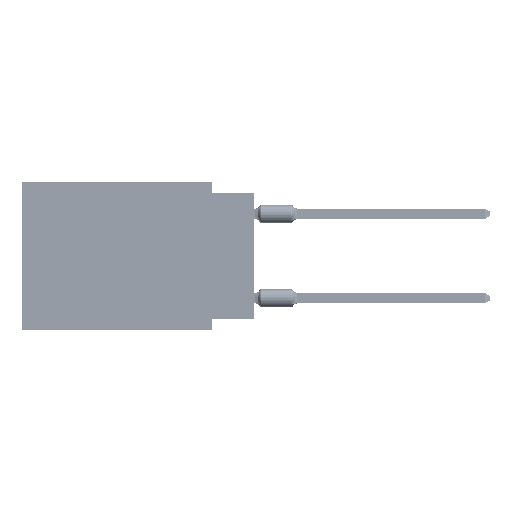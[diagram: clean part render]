
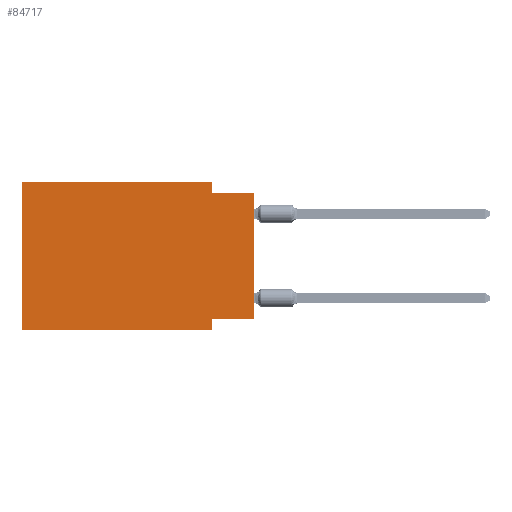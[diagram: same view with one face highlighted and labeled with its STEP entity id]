
A CAD part, left-side view. The second image highlights one B-rep face of the part: STEP entity #84717.
In plain terms, the highlighted planar face has unit normal (-1, 0, 0).
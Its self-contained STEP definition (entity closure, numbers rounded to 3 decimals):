
#614 = CARTESIAN_POINT ( 'NONE',  ( 0., 13.97, 0. ) ) ;
#1731 = DIRECTION ( 'NONE',  ( 0., 0., -1. ) ) ;
#3289 = VERTEX_POINT ( 'NONE', #62890 ) ;
#5989 = ORIENTED_EDGE ( 'NONE', *, *, #31667, .F. ) ;
#6401 = CARTESIAN_POINT ( 'NONE',  ( 0., 0., -0.635 ) ) ;
#9593 = CARTESIAN_POINT ( 'NONE',  ( 0., 0., -8.255 ) ) ;
#10153 = CARTESIAN_POINT ( 'NONE',  ( 0., 13.97, -8.89 ) ) ;
#10672 = LINE ( 'NONE', #44345, #69511 ) ;
#10804 = FACE_OUTER_BOUND ( 'NONE', #86085, .T. ) ;
#12265 = VECTOR ( 'NONE', #18580, 1000. ) ;
#14541 = EDGE_CURVE ( 'NONE', #88609, #100071, #97196, .T. ) ;
#16264 = DIRECTION ( 'NONE',  ( 0., -1., 0. ) ) ;
#18580 = DIRECTION ( 'NONE',  ( 0., -1., 0. ) ) ;
#20111 = CARTESIAN_POINT ( 'NONE',  ( 0., 0., 0. ) ) ;
#23628 = EDGE_CURVE ( 'NONE', #97169, #79795, #48381, .T. ) ;
#24776 = VECTOR ( 'NONE', #54321, 1000. ) ;
#26793 = EDGE_CURVE ( 'NONE', #40394, #40401, #34420, .T. ) ;
#26898 = ORIENTED_EDGE ( 'NONE', *, *, #90787, .F. ) ;
#27081 = ORIENTED_EDGE ( 'NONE', *, *, #23628, .T. ) ;
#31667 = EDGE_CURVE ( 'NONE', #3289, #88609, #102188, .T. ) ;
#32446 = CARTESIAN_POINT ( 'NONE',  ( 0., 2.54, -8.89 ) ) ;
#34420 = LINE ( 'NONE', #77601, #88959 ) ;
#34813 = DIRECTION ( 'NONE',  ( 0., 0., 1. ) ) ;
#35390 = CARTESIAN_POINT ( 'NONE',  ( 0., 2.54, -8.255 ) ) ;
#38254 = PLANE ( 'NONE',  #50940 ) ;
#39415 = CARTESIAN_POINT ( 'NONE',  ( 0., 13.97, -8.89 ) ) ;
#40394 = VERTEX_POINT ( 'NONE', #9593 ) ;
#40401 = VERTEX_POINT ( 'NONE', #35390 ) ;
#42485 = ORIENTED_EDGE ( 'NONE', *, *, #14541, .F. ) ;
#43152 = CARTESIAN_POINT ( 'NONE',  ( 0., 0., -0.635 ) ) ;
#43204 = VERTEX_POINT ( 'NONE', #6401 ) ;
#43496 = ORIENTED_EDGE ( 'NONE', *, *, #26793, .F. ) ;
#44345 = CARTESIAN_POINT ( 'NONE',  ( 0., 2.54, -8.89 ) ) ;
#45006 = DIRECTION ( 'NONE',  ( 0., 0., -1. ) ) ;
#46812 = EDGE_CURVE ( 'NONE', #97169, #3289, #77433, .T. ) ;
#48381 = LINE ( 'NONE', #39415, #52239 ) ;
#50940 = AXIS2_PLACEMENT_3D ( 'NONE', #55097, #97168, #45006 ) ;
#52239 = VECTOR ( 'NONE', #99429, 1000. ) ;
#54321 = DIRECTION ( 'NONE',  ( 0., 0., 1. ) ) ;
#55097 = CARTESIAN_POINT ( 'NONE',  ( 0., 13.97, 0. ) ) ;
#55126 = CARTESIAN_POINT ( 'NONE',  ( 0., 2.54, 0. ) ) ;
#61211 = CARTESIAN_POINT ( 'NONE',  ( 0., 13.97, 0. ) ) ;
#61709 = ORIENTED_EDGE ( 'NONE', *, *, #109322, .T. ) ;
#62890 = CARTESIAN_POINT ( 'NONE',  ( 0., 13.97, 0. ) ) ;
#69511 = VECTOR ( 'NONE', #1731, 1000. ) ;
#76407 = CARTESIAN_POINT ( 'NONE',  ( 0., 2.54, -0.635 ) ) ;
#77433 = LINE ( 'NONE', #614, #96973 ) ;
#77601 = CARTESIAN_POINT ( 'NONE',  ( 0., 0., -8.255 ) ) ;
#79795 = VERTEX_POINT ( 'NONE', #32446 ) ;
#81538 = VECTOR ( 'NONE', #89338, 1000. ) ;
#84717 = ADVANCED_FACE ( 'NONE', ( #10804 ), #38254, .F. ) ;
#85247 = LINE ( 'NONE', #43152, #98111 ) ;
#86028 = DIRECTION ( 'NONE',  ( 0., 1., 0. ) ) ;
#86085 = EDGE_LOOP ( 'NONE', ( #61709, #97125, #42485, #5989, #100484, #27081, #26898, #43496 ) ) ;
#88609 = VERTEX_POINT ( 'NONE', #105885 ) ;
#88959 = VECTOR ( 'NONE', #86028, 1000. ) ;
#89338 = DIRECTION ( 'NONE',  ( 0., 0., -1. ) ) ;
#90787 = EDGE_CURVE ( 'NONE', #40401, #79795, #10672, .T. ) ;
#96945 = LINE ( 'NONE', #20111, #24776 ) ;
#96973 = VECTOR ( 'NONE', #34813, 1000. ) ;
#97125 = ORIENTED_EDGE ( 'NONE', *, *, #109170, .F. ) ;
#97168 = DIRECTION ( 'NONE',  ( 1., 0., 0. ) ) ;
#97169 = VERTEX_POINT ( 'NONE', #10153 ) ;
#97196 = LINE ( 'NONE', #55126, #81538 ) ;
#98111 = VECTOR ( 'NONE', #16264, 1000. ) ;
#99429 = DIRECTION ( 'NONE',  ( 0., -1., 0. ) ) ;
#100071 = VERTEX_POINT ( 'NONE', #76407 ) ;
#100484 = ORIENTED_EDGE ( 'NONE', *, *, #46812, .F. ) ;
#102188 = LINE ( 'NONE', #61211, #12265 ) ;
#105885 = CARTESIAN_POINT ( 'NONE',  ( 0., 2.54, 0. ) ) ;
#109170 = EDGE_CURVE ( 'NONE', #100071, #43204, #85247, .T. ) ;
#109322 = EDGE_CURVE ( 'NONE', #40394, #43204, #96945, .T. ) ;
